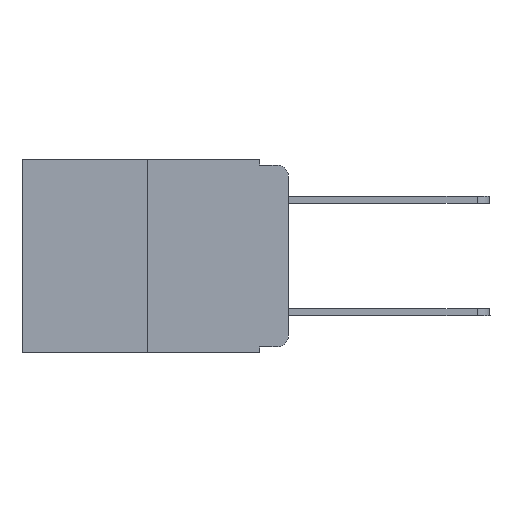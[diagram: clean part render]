
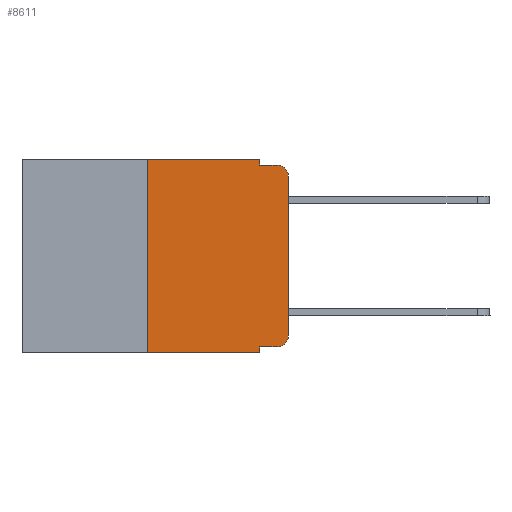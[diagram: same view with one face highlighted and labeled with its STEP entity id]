
A CAD part, left-side view. The second image highlights one B-rep face of the part: STEP entity #8611.
In plain terms, the highlighted planar face has unit normal (-1, 0, 0).
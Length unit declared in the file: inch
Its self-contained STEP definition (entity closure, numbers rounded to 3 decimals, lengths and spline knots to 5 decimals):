
#191 = CARTESIAN_POINT ( 'NONE',  ( 0., 0.051, -0.333 ) ) ;
#417 = ORIENTED_EDGE ( 'NONE', *, *, #15042, .T. ) ;
#931 = ORIENTED_EDGE ( 'NONE', *, *, #2095, .T. ) ;
#1400 = CARTESIAN_POINT ( 'NONE',  ( 0., 0., 0. ) ) ;
#1589 = VECTOR ( 'NONE', #7783, 39.37008 ) ;
#1615 = CARTESIAN_POINT ( 'NONE',  ( 0., 0.051, -0.333 ) ) ;
#2095 = EDGE_CURVE ( 'NONE', #6928, #8998, #4273, .T. ) ;
#2227 = ORIENTED_EDGE ( 'NONE', *, *, #5093, .F. ) ;
#2252 = VERTEX_POINT ( 'NONE', #6004 ) ;
#2776 = AXIS2_PLACEMENT_3D ( 'NONE', #11749, #13444, #16356 ) ;
#3037 = VECTOR ( 'NONE', #18036, 39.37008 ) ;
#3315 = CARTESIAN_POINT ( 'NONE',  ( 0., 0.473, -0.343 ) ) ;
#3317 = CIRCLE ( 'NONE', #9594, 0.02 ) ;
#3374 = CARTESIAN_POINT ( 'NONE',  ( 0., 0.473, 0. ) ) ;
#3584 = EDGE_CURVE ( 'NONE', #14395, #9860, #4972, .T. ) ;
#3615 = CARTESIAN_POINT ( 'NONE',  ( 0., 0.051, -0.343 ) ) ;
#4002 = FACE_OUTER_BOUND ( 'NONE', #19082, .T. ) ;
#4035 = LINE ( 'NONE', #17059, #1589 ) ;
#4039 = VERTEX_POINT ( 'NONE', #12717 ) ;
#4059 = CARTESIAN_POINT ( 'NONE',  ( 0., 0.051, -0.01 ) ) ;
#4231 = ORIENTED_EDGE ( 'NONE', *, *, #8565, .T. ) ;
#4273 = CIRCLE ( 'NONE', #2776, 0.02 ) ;
#4456 = VECTOR ( 'NONE', #6415, 39.37008 ) ;
#4972 = LINE ( 'NONE', #19095, #3037 ) ;
#5093 = EDGE_CURVE ( 'NONE', #9860, #8998, #17787, .T. ) ;
#5647 = CARTESIAN_POINT ( 'NONE',  ( 0., 0.25, 0. ) ) ;
#6004 = CARTESIAN_POINT ( 'NONE',  ( 0., 0., -0.313 ) ) ;
#6355 = ORIENTED_EDGE ( 'NONE', *, *, #9018, .T. ) ;
#6364 = ORIENTED_EDGE ( 'NONE', *, *, #3584, .F. ) ;
#6415 = DIRECTION ( 'NONE',  ( 0., -1., 0. ) ) ;
#6928 = VERTEX_POINT ( 'NONE', #12456 ) ;
#7253 = CARTESIAN_POINT ( 'NONE',  ( 0., 0.473, 0. ) ) ;
#7269 = VERTEX_POINT ( 'NONE', #19687 ) ;
#7707 = ORIENTED_EDGE ( 'NONE', *, *, #19438, .F. ) ;
#7783 = DIRECTION ( 'NONE',  ( 0., 0., 1. ) ) ;
#8126 = LINE ( 'NONE', #1400, #19487 ) ;
#8565 = EDGE_CURVE ( 'NONE', #17436, #4039, #8592, .T. ) ;
#8592 = LINE ( 'NONE', #191, #4456 ) ;
#8611 = ADVANCED_FACE ( 'NONE', ( #4002 ), #15946, .F. ) ;
#8880 = VERTEX_POINT ( 'NONE', #5647 ) ;
#8998 = VERTEX_POINT ( 'NONE', #13784 ) ;
#9018 = EDGE_CURVE ( 'NONE', #2252, #6928, #8126, .T. ) ;
#9594 = AXIS2_PLACEMENT_3D ( 'NONE', #17720, #12965, #19065 ) ;
#9666 = DIRECTION ( 'NONE',  ( 1., 0., 0. ) ) ;
#9860 = VERTEX_POINT ( 'NONE', #19960 ) ;
#9914 = LINE ( 'NONE', #11204, #16695 ) ;
#10600 = VERTEX_POINT ( 'NONE', #3615 ) ;
#11073 = DIRECTION ( 'NONE',  ( 0., 0., -1. ) ) ;
#11204 = CARTESIAN_POINT ( 'NONE',  ( 0., 0.051, 0. ) ) ;
#11355 = ORIENTED_EDGE ( 'NONE', *, *, #18643, .T. ) ;
#11456 = LINE ( 'NONE', #3315, #19213 ) ;
#11749 = CARTESIAN_POINT ( 'NONE',  ( 0., 0.02, -0.03 ) ) ;
#12456 = CARTESIAN_POINT ( 'NONE',  ( 0., 0., -0.03 ) ) ;
#12717 = CARTESIAN_POINT ( 'NONE',  ( 0., 0.02, -0.333 ) ) ;
#12740 = CARTESIAN_POINT ( 'NONE',  ( 0., 0.051, 0. ) ) ;
#12965 = DIRECTION ( 'NONE',  ( -1., 0., 0. ) ) ;
#13125 = EDGE_CURVE ( 'NONE', #7269, #8880, #4035, .T. ) ;
#13444 = DIRECTION ( 'NONE',  ( -1., 0., 0. ) ) ;
#13784 = CARTESIAN_POINT ( 'NONE',  ( 0., 0.02, -0.01 ) ) ;
#14141 = DIRECTION ( 'NONE',  ( 0., -1., 0. ) ) ;
#14395 = VERTEX_POINT ( 'NONE', #12740 ) ;
#14500 = AXIS2_PLACEMENT_3D ( 'NONE', #3374, #9666, #17524 ) ;
#15042 = EDGE_CURVE ( 'NONE', #7269, #10600, #11456, .T. ) ;
#15946 = PLANE ( 'NONE',  #14500 ) ;
#16356 = DIRECTION ( 'NONE',  ( 0., 0., -1. ) ) ;
#16695 = VECTOR ( 'NONE', #11073, 39.37008 ) ;
#17059 = CARTESIAN_POINT ( 'NONE',  ( 0., 0.25, 0. ) ) ;
#17436 = VERTEX_POINT ( 'NONE', #1615 ) ;
#17524 = DIRECTION ( 'NONE',  ( 0., 0., -1. ) ) ;
#17540 = EDGE_CURVE ( 'NONE', #17436, #10600, #9914, .T. ) ;
#17720 = CARTESIAN_POINT ( 'NONE',  ( 0., 0.02, -0.313 ) ) ;
#17762 = ORIENTED_EDGE ( 'NONE', *, *, #17540, .F. ) ;
#17787 = LINE ( 'NONE', #4059, #18498 ) ;
#18036 = DIRECTION ( 'NONE',  ( 0., 0., -1. ) ) ;
#18495 = ORIENTED_EDGE ( 'NONE', *, *, #13125, .F. ) ;
#18498 = VECTOR ( 'NONE', #19932, 39.37008 ) ;
#18514 = DIRECTION ( 'NONE',  ( 0., 0., 1. ) ) ;
#18543 = LINE ( 'NONE', #7253, #18790 ) ;
#18643 = EDGE_CURVE ( 'NONE', #4039, #2252, #3317, .T. ) ;
#18790 = VECTOR ( 'NONE', #19717, 39.37008 ) ;
#19065 = DIRECTION ( 'NONE',  ( 0., 0., -1. ) ) ;
#19082 = EDGE_LOOP ( 'NONE', ( #6355, #931, #2227, #6364, #7707, #18495, #417, #17762, #4231, #11355 ) ) ;
#19095 = CARTESIAN_POINT ( 'NONE',  ( 0., 0.051, 0. ) ) ;
#19213 = VECTOR ( 'NONE', #14141, 39.37008 ) ;
#19438 = EDGE_CURVE ( 'NONE', #8880, #14395, #18543, .T. ) ;
#19487 = VECTOR ( 'NONE', #18514, 39.37008 ) ;
#19687 = CARTESIAN_POINT ( 'NONE',  ( 0., 0.25, -0.343 ) ) ;
#19717 = DIRECTION ( 'NONE',  ( 0., -1., 0. ) ) ;
#19932 = DIRECTION ( 'NONE',  ( 0., -1., 0. ) ) ;
#19960 = CARTESIAN_POINT ( 'NONE',  ( 0., 0.051, -0.01 ) ) ;
